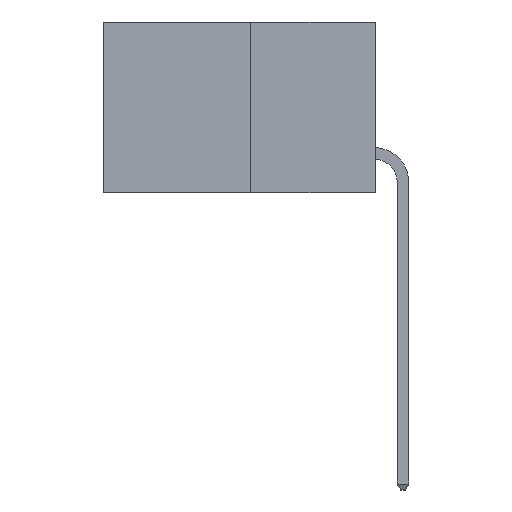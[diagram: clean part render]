
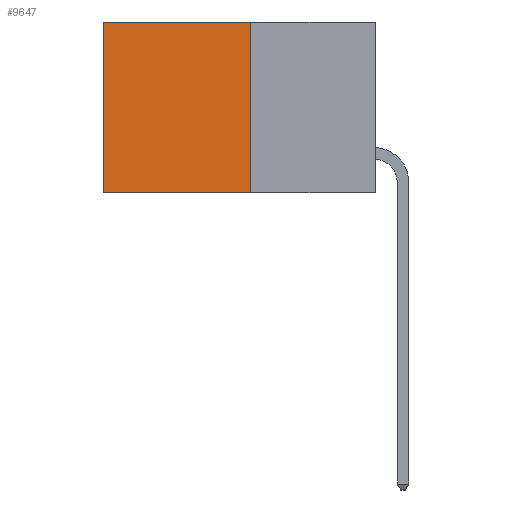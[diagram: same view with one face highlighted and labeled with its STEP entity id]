
A CAD part, left-side view. The second image highlights one B-rep face of the part: STEP entity #9647.
In plain terms, the highlighted planar face has unit normal (-1, 0, 0).
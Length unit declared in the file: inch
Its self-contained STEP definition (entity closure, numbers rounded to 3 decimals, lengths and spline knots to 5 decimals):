
#921 = ORIENTED_EDGE ( 'NONE', *, *, #12811, .F. ) ;
#1057 = DIRECTION ( 'NONE',  ( 0., 0., -1. ) ) ;
#1075 = CARTESIAN_POINT ( 'NONE',  ( 0.277, 0.59, -0.37 ) ) ;
#1574 = VECTOR ( 'NONE', #1057, 39.37008 ) ;
#2636 = VECTOR ( 'NONE', #9878, 39.37008 ) ;
#3129 = VERTEX_POINT ( 'NONE', #15320 ) ;
#3297 = VECTOR ( 'NONE', #16496, 39.37008 ) ;
#4414 = EDGE_CURVE ( 'NONE', #16381, #3129, #5538, .T. ) ;
#4944 = FACE_OUTER_BOUND ( 'NONE', #6270, .T. ) ;
#5131 = CARTESIAN_POINT ( 'NONE',  ( 0.277, 0.27, -0.37 ) ) ;
#5538 = LINE ( 'NONE', #10219, #1574 ) ;
#6168 = LINE ( 'NONE', #13693, #2636 ) ;
#6270 = EDGE_LOOP ( 'NONE', ( #11921, #921, #11073, #10351 ) ) ;
#6440 = DIRECTION ( 'NONE',  ( 0., 0., -1. ) ) ;
#6795 = LINE ( 'NONE', #1075, #3297 ) ;
#6876 = VERTEX_POINT ( 'NONE', #10739 ) ;
#9298 = DIRECTION ( 'NONE',  ( 0., 1., 0. ) ) ;
#9647 = ADVANCED_FACE ( 'NONE', ( #4944 ), #10267, .F. ) ;
#9660 = VECTOR ( 'NONE', #9298, 39.37008 ) ;
#9878 = DIRECTION ( 'NONE',  ( 0., 1., 0. ) ) ;
#10219 = CARTESIAN_POINT ( 'NONE',  ( 0.277, 0.27, -0.37 ) ) ;
#10267 = PLANE ( 'NONE',  #13082 ) ;
#10351 = ORIENTED_EDGE ( 'NONE', *, *, #10436, .T. ) ;
#10436 = EDGE_CURVE ( 'NONE', #16381, #12810, #13058, .T. ) ;
#10739 = CARTESIAN_POINT ( 'NONE',  ( 0.277, 0.59, -0.37 ) ) ;
#11073 = ORIENTED_EDGE ( 'NONE', *, *, #4414, .F. ) ;
#11719 = EDGE_CURVE ( 'NONE', #12810, #6876, #6795, .T. ) ;
#11921 = ORIENTED_EDGE ( 'NONE', *, *, #11719, .T. ) ;
#12810 = VERTEX_POINT ( 'NONE', #14968 ) ;
#12811 = EDGE_CURVE ( 'NONE', #3129, #6876, #6168, .T. ) ;
#12950 = CARTESIAN_POINT ( 'NONE',  ( 0.277, 0.27, 0. ) ) ;
#13058 = LINE ( 'NONE', #13103, #9660 ) ;
#13082 = AXIS2_PLACEMENT_3D ( 'NONE', #5131, #14134, #6440 ) ;
#13103 = CARTESIAN_POINT ( 'NONE',  ( 0.277, 0.27, 0. ) ) ;
#13693 = CARTESIAN_POINT ( 'NONE',  ( 0.277, 0.27, -0.37 ) ) ;
#14134 = DIRECTION ( 'NONE',  ( 1., 0., 0. ) ) ;
#14968 = CARTESIAN_POINT ( 'NONE',  ( 0.277, 0.59, 0. ) ) ;
#15320 = CARTESIAN_POINT ( 'NONE',  ( 0.277, 0.27, -0.37 ) ) ;
#16381 = VERTEX_POINT ( 'NONE', #12950 ) ;
#16496 = DIRECTION ( 'NONE',  ( 0., 0., -1. ) ) ;
